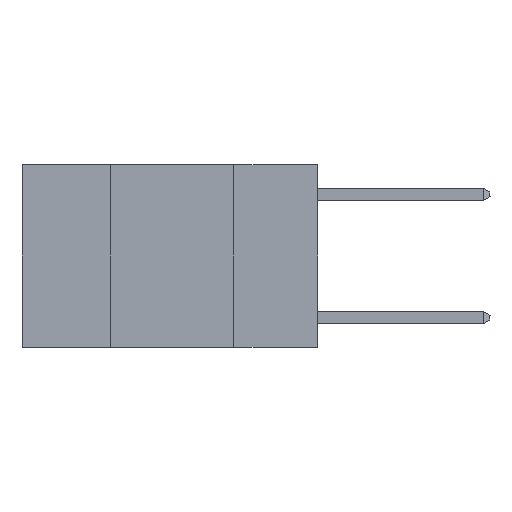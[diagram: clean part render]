
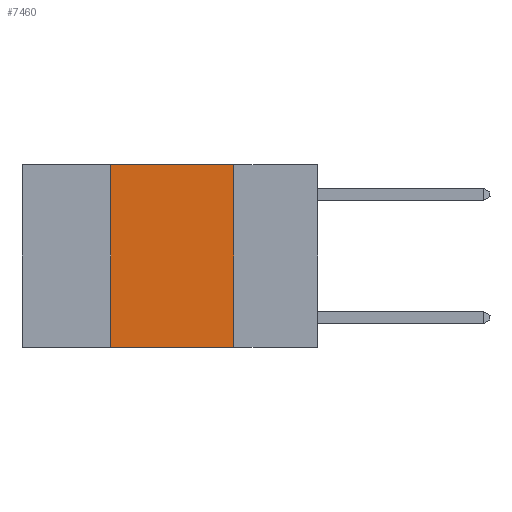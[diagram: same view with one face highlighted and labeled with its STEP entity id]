
A CAD part, left-side view. The second image highlights one B-rep face of the part: STEP entity #7460.
In plain terms, the highlighted planar face has unit normal (-1, 0, 0).
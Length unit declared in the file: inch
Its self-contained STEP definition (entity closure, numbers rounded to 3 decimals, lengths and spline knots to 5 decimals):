
#247 = LINE ( 'NONE', #5176, #10964 ) ;
#666 = EDGE_CURVE ( 'NONE', #3614, #4379, #9893, .T. ) ;
#1423 = DIRECTION ( 'NONE',  ( 0., 0., 1. ) ) ;
#1557 = ORIENTED_EDGE ( 'NONE', *, *, #5842, .F. ) ;
#2256 = CARTESIAN_POINT ( 'NONE',  ( 0., 0.17, 0. ) ) ;
#2316 = LINE ( 'NONE', #2468, #9292 ) ;
#2339 = EDGE_CURVE ( 'NONE', #12388, #6804, #247, .T. ) ;
#2468 = CARTESIAN_POINT ( 'NONE',  ( 0., 0.17, 0. ) ) ;
#2646 = CARTESIAN_POINT ( 'NONE',  ( 0., 0.42, 0. ) ) ;
#2925 = EDGE_CURVE ( 'NONE', #3614, #12388, #13571, .T. ) ;
#3343 = CARTESIAN_POINT ( 'NONE',  ( 0., 0.42, -0.37 ) ) ;
#3614 = VERTEX_POINT ( 'NONE', #3343 ) ;
#3816 = DIRECTION ( 'NONE',  ( 0., 0., -1. ) ) ;
#4379 = VERTEX_POINT ( 'NONE', #13814 ) ;
#4409 = CARTESIAN_POINT ( 'NONE',  ( 0., 0.42, 0. ) ) ;
#5122 = CARTESIAN_POINT ( 'NONE',  ( 0., 0.6, 0. ) ) ;
#5176 = CARTESIAN_POINT ( 'NONE',  ( 0., 0.6, 0. ) ) ;
#5347 = CARTESIAN_POINT ( 'NONE',  ( 0., 0.6, -0.37 ) ) ;
#5842 = EDGE_CURVE ( 'NONE', #6804, #4379, #2316, .T. ) ;
#6416 = VECTOR ( 'NONE', #1423, 39.37008 ) ;
#6804 = VERTEX_POINT ( 'NONE', #2256 ) ;
#7201 = DIRECTION ( 'NONE',  ( 0., 0., -1. ) ) ;
#7460 = ADVANCED_FACE ( 'NONE', ( #13779 ), #10058, .F. ) ;
#7526 = ORIENTED_EDGE ( 'NONE', *, *, #2925, .F. ) ;
#7621 = AXIS2_PLACEMENT_3D ( 'NONE', #5122, #14925, #3816 ) ;
#9292 = VECTOR ( 'NONE', #7201, 39.37008 ) ;
#9409 = EDGE_LOOP ( 'NONE', ( #1557, #14186, #7526, #14572 ) ) ;
#9541 = VECTOR ( 'NONE', #14909, 39.37008 ) ;
#9893 = LINE ( 'NONE', #5347, #9541 ) ;
#10058 = PLANE ( 'NONE',  #7621 ) ;
#10964 = VECTOR ( 'NONE', #13518, 39.37008 ) ;
#12388 = VERTEX_POINT ( 'NONE', #4409 ) ;
#13518 = DIRECTION ( 'NONE',  ( 0., -1., 0. ) ) ;
#13571 = LINE ( 'NONE', #2646, #6416 ) ;
#13779 = FACE_OUTER_BOUND ( 'NONE', #9409, .T. ) ;
#13814 = CARTESIAN_POINT ( 'NONE',  ( 0., 0.17, -0.37 ) ) ;
#14186 = ORIENTED_EDGE ( 'NONE', *, *, #2339, .F. ) ;
#14572 = ORIENTED_EDGE ( 'NONE', *, *, #666, .T. ) ;
#14909 = DIRECTION ( 'NONE',  ( 0., -1., 0. ) ) ;
#14925 = DIRECTION ( 'NONE',  ( 1., 0., 0. ) ) ;
